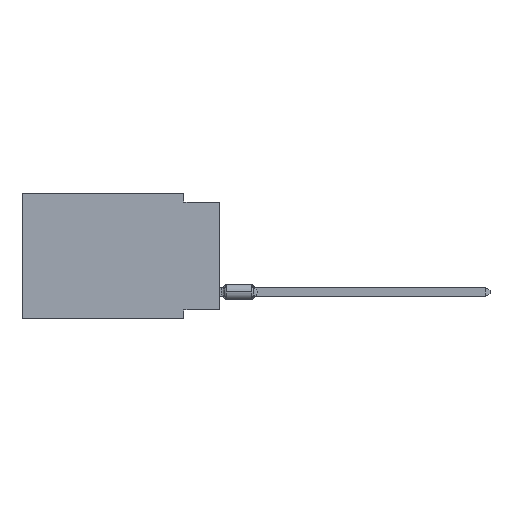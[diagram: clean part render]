
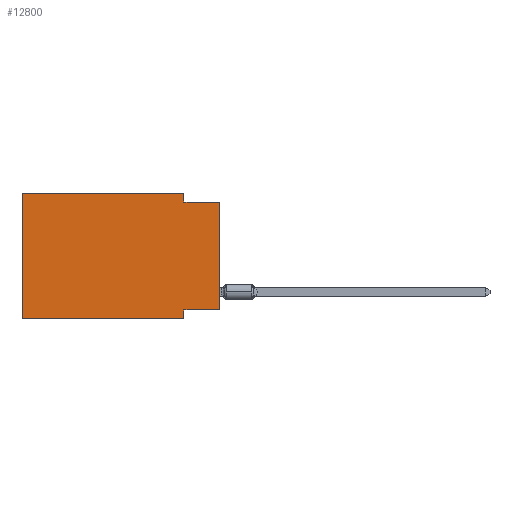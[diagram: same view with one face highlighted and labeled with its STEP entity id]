
A CAD part, left-side view. The second image highlights one B-rep face of the part: STEP entity #12800.
In plain terms, the highlighted planar face has unit normal (-1, 0, 0).
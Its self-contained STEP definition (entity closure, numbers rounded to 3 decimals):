
#234 = CARTESIAN_POINT ( 'NONE',  ( 0., 2.54, -0.635 ) ) ;
#1297 = CARTESIAN_POINT ( 'NONE',  ( 0., 13.97, -8.89 ) ) ;
#2531 = DIRECTION ( 'NONE',  ( 0., 0., 1. ) ) ;
#3180 = LINE ( 'NONE', #21364, #19868 ) ;
#4270 = VERTEX_POINT ( 'NONE', #234 ) ;
#4839 = CARTESIAN_POINT ( 'NONE',  ( 0., 0., -0.635 ) ) ;
#5474 = LINE ( 'NONE', #14726, #11116 ) ;
#5534 = VERTEX_POINT ( 'NONE', #14029 ) ;
#5751 = PLANE ( 'NONE',  #5831 ) ;
#5831 = AXIS2_PLACEMENT_3D ( 'NONE', #7881, #10462, #17417 ) ;
#6810 = VECTOR ( 'NONE', #23907, 1000. ) ;
#7350 = LINE ( 'NONE', #9933, #14617 ) ;
#7453 = ORIENTED_EDGE ( 'NONE', *, *, #11152, .F. ) ;
#7831 = DIRECTION ( 'NONE',  ( 0., -1., 0. ) ) ;
#7881 = CARTESIAN_POINT ( 'NONE',  ( 0., 13.97, 0. ) ) ;
#9492 = EDGE_CURVE ( 'NONE', #14419, #21965, #28873, .T. ) ;
#9933 = CARTESIAN_POINT ( 'NONE',  ( 0., 0., 0. ) ) ;
#10150 = CARTESIAN_POINT ( 'NONE',  ( 0., 2.54, 0. ) ) ;
#10462 = DIRECTION ( 'NONE',  ( 1., 0., 0. ) ) ;
#10878 = CARTESIAN_POINT ( 'NONE',  ( 0., 2.54, -8.89 ) ) ;
#11116 = VECTOR ( 'NONE', #23947, 1000. ) ;
#11152 = EDGE_CURVE ( 'NONE', #4270, #21698, #16074, .T. ) ;
#12654 = EDGE_CURVE ( 'NONE', #22258, #14384, #3180, .T. ) ;
#12800 = ADVANCED_FACE ( 'NONE', ( #26790 ), #5751, .F. ) ;
#12803 = VECTOR ( 'NONE', #7831, 1000. ) ;
#13030 = ORIENTED_EDGE ( 'NONE', *, *, #29560, .F. ) ;
#13117 = CARTESIAN_POINT ( 'NONE',  ( 0., 2.54, -8.89 ) ) ;
#13421 = LINE ( 'NONE', #13117, #22994 ) ;
#13465 = LINE ( 'NONE', #25553, #27317 ) ;
#13521 = ORIENTED_EDGE ( 'NONE', *, *, #18111, .F. ) ;
#13710 = DIRECTION ( 'NONE',  ( 0., 0., -1. ) ) ;
#14029 = CARTESIAN_POINT ( 'NONE',  ( 0., 2.54, 0. ) ) ;
#14384 = VERTEX_POINT ( 'NONE', #27484 ) ;
#14419 = VERTEX_POINT ( 'NONE', #26254 ) ;
#14617 = VECTOR ( 'NONE', #21575, 1000. ) ;
#14726 = CARTESIAN_POINT ( 'NONE',  ( 0., 13.97, 0. ) ) ;
#15702 = EDGE_CURVE ( 'NONE', #22258, #21698, #7350, .T. ) ;
#16074 = LINE ( 'NONE', #20775, #24442 ) ;
#17039 = EDGE_LOOP ( 'NONE', ( #29086, #7453, #13030, #23635, #13521, #28698, #28583, #23495 ) ) ;
#17217 = CARTESIAN_POINT ( 'NONE',  ( 0., 0., -8.255 ) ) ;
#17417 = DIRECTION ( 'NONE',  ( 0., 0., -1. ) ) ;
#17986 = VERTEX_POINT ( 'NONE', #20128 ) ;
#18111 = EDGE_CURVE ( 'NONE', #14419, #17986, #13465, .T. ) ;
#19868 = VECTOR ( 'NONE', #21514, 1000. ) ;
#20128 = CARTESIAN_POINT ( 'NONE',  ( 0., 13.97, 0. ) ) ;
#20775 = CARTESIAN_POINT ( 'NONE',  ( 0., 0., -0.635 ) ) ;
#21364 = CARTESIAN_POINT ( 'NONE',  ( 0., 0., -8.255 ) ) ;
#21514 = DIRECTION ( 'NONE',  ( 0., 1., 0. ) ) ;
#21575 = DIRECTION ( 'NONE',  ( 0., 0., 1. ) ) ;
#21698 = VERTEX_POINT ( 'NONE', #4839 ) ;
#21965 = VERTEX_POINT ( 'NONE', #10878 ) ;
#22258 = VERTEX_POINT ( 'NONE', #17217 ) ;
#22383 = EDGE_CURVE ( 'NONE', #14384, #21965, #13421, .T. ) ;
#22994 = VECTOR ( 'NONE', #13710, 1000. ) ;
#23495 = ORIENTED_EDGE ( 'NONE', *, *, #12654, .F. ) ;
#23635 = ORIENTED_EDGE ( 'NONE', *, *, #24424, .F. ) ;
#23907 = DIRECTION ( 'NONE',  ( 0., 0., -1. ) ) ;
#23947 = DIRECTION ( 'NONE',  ( 0., -1., 0. ) ) ;
#24199 = LINE ( 'NONE', #10150, #6810 ) ;
#24424 = EDGE_CURVE ( 'NONE', #17986, #5534, #5474, .T. ) ;
#24442 = VECTOR ( 'NONE', #25300, 1000. ) ;
#25300 = DIRECTION ( 'NONE',  ( 0., -1., 0. ) ) ;
#25553 = CARTESIAN_POINT ( 'NONE',  ( 0., 13.97, 0. ) ) ;
#26254 = CARTESIAN_POINT ( 'NONE',  ( 0., 13.97, -8.89 ) ) ;
#26790 = FACE_OUTER_BOUND ( 'NONE', #17039, .T. ) ;
#27317 = VECTOR ( 'NONE', #2531, 1000. ) ;
#27484 = CARTESIAN_POINT ( 'NONE',  ( 0., 2.54, -8.255 ) ) ;
#28583 = ORIENTED_EDGE ( 'NONE', *, *, #22383, .F. ) ;
#28698 = ORIENTED_EDGE ( 'NONE', *, *, #9492, .T. ) ;
#28873 = LINE ( 'NONE', #1297, #12803 ) ;
#29086 = ORIENTED_EDGE ( 'NONE', *, *, #15702, .T. ) ;
#29560 = EDGE_CURVE ( 'NONE', #5534, #4270, #24199, .T. ) ;
